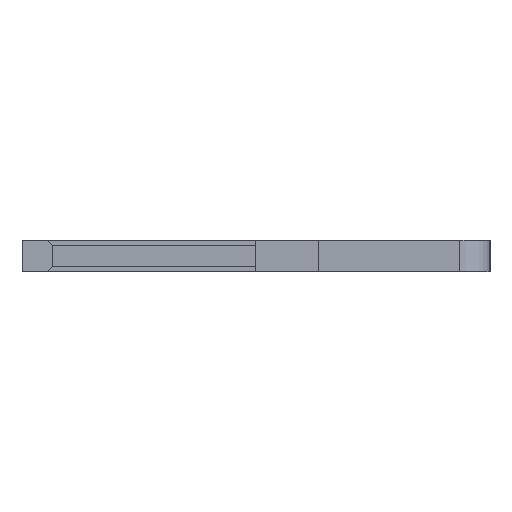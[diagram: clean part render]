
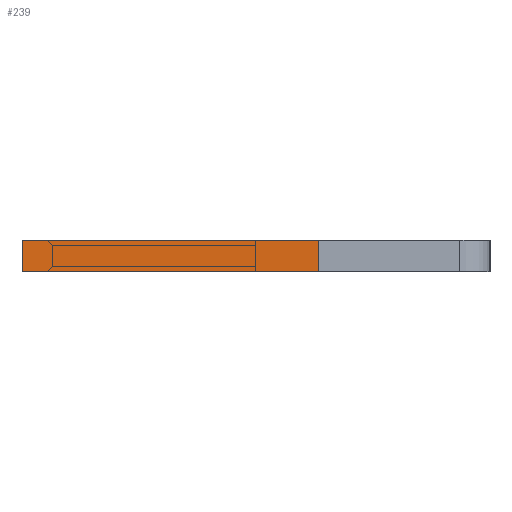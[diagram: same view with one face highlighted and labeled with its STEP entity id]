
A CAD part, left-side view. The second image highlights one B-rep face of the part: STEP entity #239.
In plain terms, the highlighted face is planar.
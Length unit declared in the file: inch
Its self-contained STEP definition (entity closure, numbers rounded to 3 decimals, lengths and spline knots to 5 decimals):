
#92 = EDGE_CURVE ( 'NONE', #652, #153, #2376, .T. ) ;
#153 = VERTEX_POINT ( 'NONE', #2572 ) ;
#239 = ADVANCED_FACE ( 'NONE', ( #682 ), #4335, .F. ) ;
#447 = CARTESIAN_POINT ( 'NONE',  ( -0.01, 0.15, -0.04 ) ) ;
#469 = CARTESIAN_POINT ( 'NONE',  ( -0.01, -0.04, -0.04 ) ) ;
#484 = DIRECTION ( 'NONE',  ( 1., 0., 0. ) ) ;
#616 = VERTEX_POINT ( 'NONE', #469 ) ;
#652 = VERTEX_POINT ( 'NONE', #1910 ) ;
#682 = FACE_OUTER_BOUND ( 'NONE', #2249, .T. ) ;
#923 = EDGE_CURVE ( 'NONE', #616, #2266, #2754, .T. ) ;
#929 = CARTESIAN_POINT ( 'NONE',  ( -0.01, 0.15, -0.04 ) ) ;
#1061 = ORIENTED_EDGE ( 'NONE', *, *, #923, .T. ) ;
#1228 = VECTOR ( 'NONE', #3614, 39.37008 ) ;
#1248 = EDGE_CURVE ( 'NONE', #153, #2266, #3126, .T. ) ;
#1269 = VECTOR ( 'NONE', #2706, 39.37008 ) ;
#1400 = ORIENTED_EDGE ( 'NONE', *, *, #92, .F. ) ;
#1600 = ORIENTED_EDGE ( 'NONE', *, *, #1248, .F. ) ;
#1698 = LINE ( 'NONE', #3054, #2981 ) ;
#1840 = CARTESIAN_POINT ( 'NONE',  ( 0.01, 0.15, -0.04 ) ) ;
#1910 = CARTESIAN_POINT ( 'NONE',  ( 0.01, -0.04, -0.04 ) ) ;
#2194 = DIRECTION ( 'NONE',  ( 0., 0., 1. ) ) ;
#2249 = EDGE_LOOP ( 'NONE', ( #1061, #1600, #1400, #2495 ) ) ;
#2266 = VERTEX_POINT ( 'NONE', #929 ) ;
#2376 = LINE ( 'NONE', #3651, #1228 ) ;
#2381 = DIRECTION ( 'NONE',  ( -1., 0., 0. ) ) ;
#2495 = ORIENTED_EDGE ( 'NONE', *, *, #2624, .T. ) ;
#2572 = CARTESIAN_POINT ( 'NONE',  ( 0.01, 0.15, -0.04 ) ) ;
#2617 = DIRECTION ( 'NONE',  ( 0., 1., 0. ) ) ;
#2624 = EDGE_CURVE ( 'NONE', #652, #616, #1698, .T. ) ;
#2706 = DIRECTION ( 'NONE',  ( -1., 0., 0. ) ) ;
#2754 = LINE ( 'NONE', #447, #3588 ) ;
#2981 = VECTOR ( 'NONE', #2381, 39.37008 ) ;
#3054 = CARTESIAN_POINT ( 'NONE',  ( 0.01, -0.04, -0.04 ) ) ;
#3126 = LINE ( 'NONE', #3776, #1269 ) ;
#3315 = AXIS2_PLACEMENT_3D ( 'NONE', #1840, #2194, #484 ) ;
#3588 = VECTOR ( 'NONE', #2617, 39.37008 ) ;
#3614 = DIRECTION ( 'NONE',  ( 0., 1., 0. ) ) ;
#3651 = CARTESIAN_POINT ( 'NONE',  ( 0.01, 0.15, -0.04 ) ) ;
#3776 = CARTESIAN_POINT ( 'NONE',  ( 0.01, 0.15, -0.04 ) ) ;
#4335 = PLANE ( 'NONE',  #3315 ) ;
